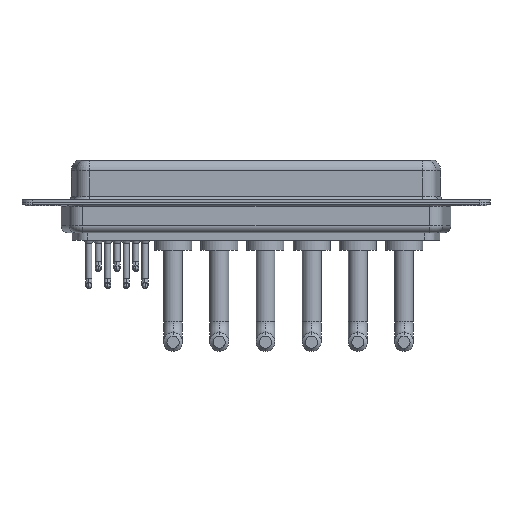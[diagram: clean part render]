
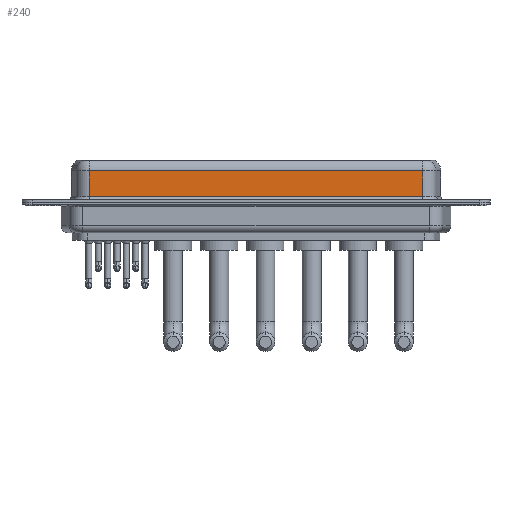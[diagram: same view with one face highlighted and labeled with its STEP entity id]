
A CAD part, front view. The second image highlights one B-rep face of the part: STEP entity #240.
In plain terms, the highlighted planar face has unit normal (0, -1, 0).
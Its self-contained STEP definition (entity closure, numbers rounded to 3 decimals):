
#240 = ADVANCED_FACE ( 'NONE', ( #2064 ), #11222, .F. ) ;
#349 = CARTESIAN_POINT ( 'NONE',  ( 7.038, -3.95, 4.65 ) ) ;
#908 = DIRECTION ( 'NONE',  ( 0., 1., 0. ) ) ;
#1079 = CARTESIAN_POINT ( 'NONE',  ( 56.462, -3.95, 6.4 ) ) ;
#1288 = AXIS2_PLACEMENT_3D ( 'NONE', #7374, #908, #8615 ) ;
#1412 = EDGE_CURVE ( 'NONE', #4100, #12793, #5673, .T. ) ;
#1723 = ORIENTED_EDGE ( 'NONE', *, *, #14522, .T. ) ;
#2064 = FACE_OUTER_BOUND ( 'NONE', #13832, .T. ) ;
#2238 = ORIENTED_EDGE ( 'NONE', *, *, #15412, .F. ) ;
#2360 = CARTESIAN_POINT ( 'NONE',  ( 56.462, -3.95, 4.65 ) ) ;
#4100 = VERTEX_POINT ( 'NONE', #16186 ) ;
#4546 = VECTOR ( 'NONE', #8452, 1000. ) ;
#5011 = CARTESIAN_POINT ( 'NONE',  ( 56.462, -3.95, 4.65 ) ) ;
#5147 = CARTESIAN_POINT ( 'NONE',  ( 56.462, -3.95, 0.9 ) ) ;
#5673 = LINE ( 'NONE', #7822, #8653 ) ;
#7374 = CARTESIAN_POINT ( 'NONE',  ( 56.462, -3.95, 6.4 ) ) ;
#7822 = CARTESIAN_POINT ( 'NONE',  ( 56.462, -3.95, 0.9 ) ) ;
#8452 = DIRECTION ( 'NONE',  ( 0., 0., -1. ) ) ;
#8615 = DIRECTION ( 'NONE',  ( 0., 0., 1. ) ) ;
#8653 = VECTOR ( 'NONE', #15558, 1000. ) ;
#9639 = EDGE_CURVE ( 'NONE', #10333, #4100, #12648, .T. ) ;
#9885 = VECTOR ( 'NONE', #12619, 1000. ) ;
#9955 = CARTESIAN_POINT ( 'NONE',  ( 7.038, -3.95, 6.4 ) ) ;
#10333 = VERTEX_POINT ( 'NONE', #349 ) ;
#11222 = PLANE ( 'NONE',  #1288 ) ;
#12566 = DIRECTION ( 'NONE',  ( 0., 0., -1. ) ) ;
#12606 = ORIENTED_EDGE ( 'NONE', *, *, #1412, .T. ) ;
#12619 = DIRECTION ( 'NONE',  ( -1., 0., 0. ) ) ;
#12648 = LINE ( 'NONE', #9955, #15136 ) ;
#12793 = VERTEX_POINT ( 'NONE', #5147 ) ;
#13832 = EDGE_LOOP ( 'NONE', ( #2238, #1723, #14595, #12606 ) ) ;
#13841 = LINE ( 'NONE', #1079, #4546 ) ;
#13877 = LINE ( 'NONE', #2360, #9885 ) ;
#14522 = EDGE_CURVE ( 'NONE', #15629, #10333, #13877, .T. ) ;
#14595 = ORIENTED_EDGE ( 'NONE', *, *, #9639, .T. ) ;
#15136 = VECTOR ( 'NONE', #12566, 1000. ) ;
#15412 = EDGE_CURVE ( 'NONE', #15629, #12793, #13841, .T. ) ;
#15558 = DIRECTION ( 'NONE',  ( 1., 0., 0. ) ) ;
#15629 = VERTEX_POINT ( 'NONE', #5011 ) ;
#16186 = CARTESIAN_POINT ( 'NONE',  ( 7.038, -3.95, 0.9 ) ) ;
